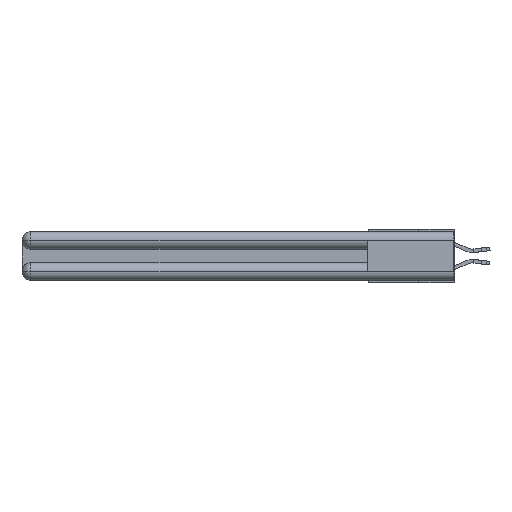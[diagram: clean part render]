
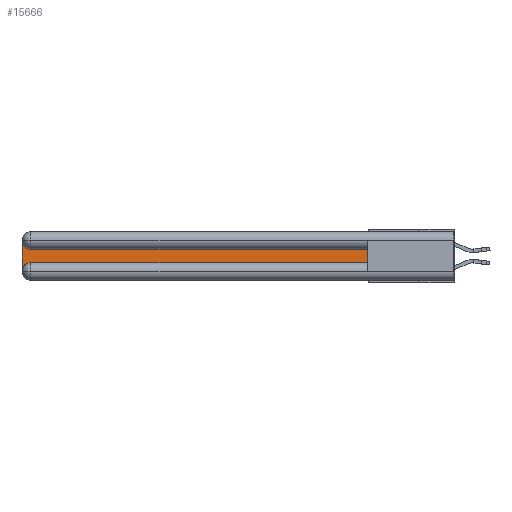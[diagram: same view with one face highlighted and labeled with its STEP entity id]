
A CAD part, left-side view. The second image highlights one B-rep face of the part: STEP entity #15666.
In plain terms, the highlighted planar face has unit normal (-1, 0, 0).
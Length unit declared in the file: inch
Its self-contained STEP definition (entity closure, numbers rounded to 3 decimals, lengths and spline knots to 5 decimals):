
#516 = CARTESIAN_POINT ( 'NONE',  ( 0.075, 3., -0.2775 ) ) ;
#1128 = EDGE_CURVE ( 'NONE', #27604, #26585, #3957, .T. ) ;
#1255 = CIRCLE ( 'NONE', #19180, 0.06 ) ;
#3286 = VECTOR ( 'NONE', #22843, 39.37008 ) ;
#3957 = LINE ( 'NONE', #7746, #3286 ) ;
#4145 = ORIENTED_EDGE ( 'NONE', *, *, #6001, .T. ) ;
#4827 = VECTOR ( 'NONE', #24937, 39.37008 ) ;
#5349 = CARTESIAN_POINT ( 'NONE',  ( 0.075, 0.6, -0.1225 ) ) ;
#5427 = ORIENTED_EDGE ( 'NONE', *, *, #8059, .T. ) ;
#6001 = EDGE_CURVE ( 'NONE', #11889, #7185, #1255, .T. ) ;
#6860 = EDGE_CURVE ( 'NONE', #13699, #27604, #7882, .T. ) ;
#7185 = VERTEX_POINT ( 'NONE', #8398 ) ;
#7211 = VECTOR ( 'NONE', #16287, 39.37008 ) ;
#7458 = DIRECTION ( 'NONE',  ( 1., 0., 0. ) ) ;
#7507 = ORIENTED_EDGE ( 'NONE', *, *, #1128, .T. ) ;
#7746 = CARTESIAN_POINT ( 'NONE',  ( 0.075, 0.6, -0.2175 ) ) ;
#7882 = LINE ( 'NONE', #13716, #7211 ) ;
#7925 = CARTESIAN_POINT ( 'NONE',  ( 0.075, 2.94, -0.1225 ) ) ;
#8059 = EDGE_CURVE ( 'NONE', #7185, #14733, #20551, .T. ) ;
#8398 = CARTESIAN_POINT ( 'NONE',  ( 0.075, 3., -0.0625 ) ) ;
#9356 = LINE ( 'NONE', #5349, #25432 ) ;
#9622 = CARTESIAN_POINT ( 'NONE',  ( 0.075, 3., -0.1225 ) ) ;
#10013 = CIRCLE ( 'NONE', #13580, 0.06 ) ;
#11354 = FACE_OUTER_BOUND ( 'NONE', #24890, .T. ) ;
#11779 = ORIENTED_EDGE ( 'NONE', *, *, #25715, .T. ) ;
#11802 = CARTESIAN_POINT ( 'NONE',  ( 0.075, 2.94, -0.2775 ) ) ;
#11889 = VERTEX_POINT ( 'NONE', #7925 ) ;
#12888 = CARTESIAN_POINT ( 'NONE',  ( 0.075, 0.6, -0.1225 ) ) ;
#13580 = AXIS2_PLACEMENT_3D ( 'NONE', #11802, #20404, #16164 ) ;
#13699 = VERTEX_POINT ( 'NONE', #21910 ) ;
#13716 = CARTESIAN_POINT ( 'NONE',  ( 0.075, 0.6, -0.2175 ) ) ;
#14229 = CARTESIAN_POINT ( 'NONE',  ( 0.075, 0.6, -0.2175 ) ) ;
#14483 = DIRECTION ( 'NONE',  ( 1., 0., 0. ) ) ;
#14733 = VERTEX_POINT ( 'NONE', #516 ) ;
#15666 = ADVANCED_FACE ( 'NONE', ( #11354 ), #20015, .F. ) ;
#16164 = DIRECTION ( 'NONE',  ( 0., 0., -1. ) ) ;
#16287 = DIRECTION ( 'NONE',  ( 0., -1., 0. ) ) ;
#18410 = DIRECTION ( 'NONE',  ( 0., 0., -1. ) ) ;
#18968 = AXIS2_PLACEMENT_3D ( 'NONE', #9622, #7458, #22375 ) ;
#19180 = AXIS2_PLACEMENT_3D ( 'NONE', #27017, #14483, #18410 ) ;
#20015 = PLANE ( 'NONE',  #18968 ) ;
#20217 = DIRECTION ( 'NONE',  ( 0., 1., 0. ) ) ;
#20404 = DIRECTION ( 'NONE',  ( 1., 0., 0. ) ) ;
#20551 = LINE ( 'NONE', #24757, #4827 ) ;
#20559 = ORIENTED_EDGE ( 'NONE', *, *, #21388, .T. ) ;
#21388 = EDGE_CURVE ( 'NONE', #26585, #11889, #9356, .T. ) ;
#21910 = CARTESIAN_POINT ( 'NONE',  ( 0.075, 2.94, -0.2175 ) ) ;
#22375 = DIRECTION ( 'NONE',  ( 0., 0., -1. ) ) ;
#22843 = DIRECTION ( 'NONE',  ( 0., 0., 1. ) ) ;
#22916 = ORIENTED_EDGE ( 'NONE', *, *, #6860, .T. ) ;
#24757 = CARTESIAN_POINT ( 'NONE',  ( 0.075, 3., -0.2175 ) ) ;
#24890 = EDGE_LOOP ( 'NONE', ( #20559, #4145, #5427, #11779, #22916, #7507 ) ) ;
#24937 = DIRECTION ( 'NONE',  ( 0., 0., -1. ) ) ;
#25432 = VECTOR ( 'NONE', #20217, 39.37008 ) ;
#25715 = EDGE_CURVE ( 'NONE', #14733, #13699, #10013, .T. ) ;
#26585 = VERTEX_POINT ( 'NONE', #12888 ) ;
#27017 = CARTESIAN_POINT ( 'NONE',  ( 0.075, 2.94, -0.0625 ) ) ;
#27604 = VERTEX_POINT ( 'NONE', #14229 ) ;
